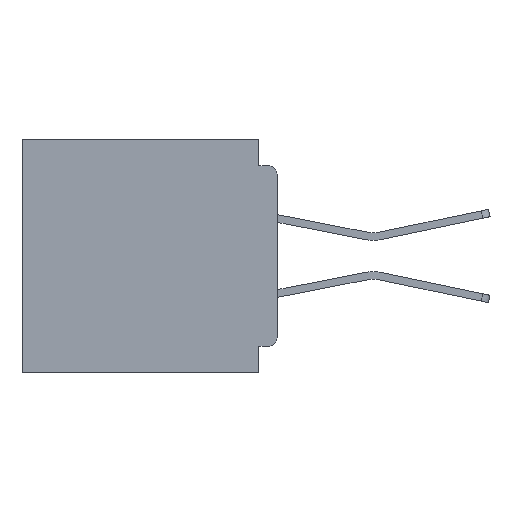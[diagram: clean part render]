
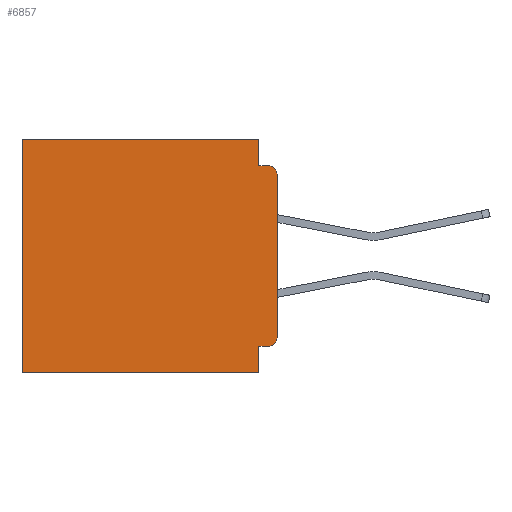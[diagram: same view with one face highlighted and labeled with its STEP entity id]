
A CAD part, left-side view. The second image highlights one B-rep face of the part: STEP entity #6857.
In plain terms, the highlighted planar face has unit normal (-1, 0, 0).
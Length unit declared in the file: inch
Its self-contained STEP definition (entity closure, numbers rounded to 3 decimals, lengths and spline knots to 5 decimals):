
#730 = LINE ( 'NONE', #44997, #26693 ) ;
#810 = VERTEX_POINT ( 'NONE', #28560 ) ;
#841 = EDGE_CURVE ( 'NONE', #22364, #8738, #36034, .T. ) ;
#1111 = AXIS2_PLACEMENT_3D ( 'NONE', #43485, #5299, #29916 ) ;
#1698 = ORIENTED_EDGE ( 'NONE', *, *, #16101, .T. ) ;
#1900 = DIRECTION ( 'NONE',  ( 0., 1., 0. ) ) ;
#2054 = CARTESIAN_POINT ( 'NONE',  ( 0.3, 0.031, 0. ) ) ;
#2116 = EDGE_CURVE ( 'NONE', #8738, #43184, #38074, .T. ) ;
#2700 = LINE ( 'NONE', #23927, #32981 ) ;
#2707 = DIRECTION ( 'NONE',  ( 0., 0., -1. ) ) ;
#3370 = CARTESIAN_POINT ( 'NONE',  ( 0.3, 0.031, -0.355 ) ) ;
#4194 = VERTEX_POINT ( 'NONE', #29689 ) ;
#4697 = VERTEX_POINT ( 'NONE', #42580 ) ;
#5299 = DIRECTION ( 'NONE',  ( 1., 0., 0. ) ) ;
#6207 = ORIENTED_EDGE ( 'NONE', *, *, #26114, .T. ) ;
#6353 = EDGE_CURVE ( 'NONE', #810, #29096, #37275, .T. ) ;
#6642 = EDGE_CURVE ( 'NONE', #4697, #36173, #26437, .T. ) ;
#6857 = ADVANCED_FACE ( 'NONE', ( #16553 ), #26431, .F. ) ;
#7925 = DIRECTION ( 'NONE',  ( 0., 0., -1. ) ) ;
#8738 = VERTEX_POINT ( 'NONE', #25829 ) ;
#8874 = CARTESIAN_POINT ( 'NONE',  ( 0.3, 0.015, -0.06 ) ) ;
#9277 = EDGE_CURVE ( 'NONE', #29096, #4697, #17986, .T. ) ;
#9750 = CARTESIAN_POINT ( 'NONE',  ( 0.3, 0.015, -0.34 ) ) ;
#10229 = ORIENTED_EDGE ( 'NONE', *, *, #28283, .F. ) ;
#10292 = DIRECTION ( 'NONE',  ( 0., 1., 0. ) ) ;
#12437 = DIRECTION ( 'NONE',  ( 0., 0., -1. ) ) ;
#13317 = DIRECTION ( 'NONE',  ( 0., 0., -1. ) ) ;
#15151 = VECTOR ( 'NONE', #23886, 39.37008 ) ;
#15288 = CARTESIAN_POINT ( 'NONE',  ( 0.3, 0.437, 0. ) ) ;
#16058 = CARTESIAN_POINT ( 'NONE',  ( 0.3, 0., -0.355 ) ) ;
#16101 = EDGE_CURVE ( 'NONE', #22364, #39197, #730, .T. ) ;
#16553 = FACE_OUTER_BOUND ( 'NONE', #22328, .T. ) ;
#17986 = LINE ( 'NONE', #32623, #27230 ) ;
#18649 = VECTOR ( 'NONE', #29374, 39.37008 ) ;
#18813 = VECTOR ( 'NONE', #1900, 39.37008 ) ;
#18898 = CARTESIAN_POINT ( 'NONE',  ( 0.3, 0.437, -0.4 ) ) ;
#19289 = AXIS2_PLACEMENT_3D ( 'NONE', #8874, #33376, #12437 ) ;
#19544 = ORIENTED_EDGE ( 'NONE', *, *, #841, .F. ) ;
#22328 = EDGE_LOOP ( 'NONE', ( #10229, #6207, #41476, #19544, #1698, #33990, #35328, #25361, #26263, #43523 ) ) ;
#22364 = VERTEX_POINT ( 'NONE', #30848 ) ;
#23886 = DIRECTION ( 'NONE',  ( 0., 0., -1. ) ) ;
#23927 = CARTESIAN_POINT ( 'NONE',  ( 0.3, 0.437, -0.4 ) ) ;
#25361 = ORIENTED_EDGE ( 'NONE', *, *, #9277, .F. ) ;
#25603 = LINE ( 'NONE', #41133, #15151 ) ;
#25829 = CARTESIAN_POINT ( 'NONE',  ( 0.3, 0.031, -0.045 ) ) ;
#26114 = EDGE_CURVE ( 'NONE', #42092, #43184, #34357, .T. ) ;
#26263 = ORIENTED_EDGE ( 'NONE', *, *, #6353, .F. ) ;
#26431 = PLANE ( 'NONE',  #1111 ) ;
#26437 = LINE ( 'NONE', #38382, #34514 ) ;
#26693 = VECTOR ( 'NONE', #10292, 39.37008 ) ;
#26800 = DIRECTION ( 'NONE',  ( 0., -1., 0. ) ) ;
#27230 = VECTOR ( 'NONE', #7925, 39.37008 ) ;
#28283 = EDGE_CURVE ( 'NONE', #42092, #4194, #25603, .T. ) ;
#28560 = CARTESIAN_POINT ( 'NONE',  ( 0.3, 0.015, -0.355 ) ) ;
#28895 = VECTOR ( 'NONE', #26800, 39.37008 ) ;
#28956 = EDGE_CURVE ( 'NONE', #810, #4194, #35257, .T. ) ;
#29096 = VERTEX_POINT ( 'NONE', #3370 ) ;
#29374 = DIRECTION ( 'NONE',  ( 0., 0., -1. ) ) ;
#29689 = CARTESIAN_POINT ( 'NONE',  ( 0.3, 0., -0.34 ) ) ;
#29916 = DIRECTION ( 'NONE',  ( 0., 0., -1. ) ) ;
#30282 = EDGE_CURVE ( 'NONE', #39197, #36173, #2700, .T. ) ;
#30848 = CARTESIAN_POINT ( 'NONE',  ( 0.3, 0.031, 0. ) ) ;
#32623 = CARTESIAN_POINT ( 'NONE',  ( 0.3, 0.031, -0.4 ) ) ;
#32981 = VECTOR ( 'NONE', #2707, 39.37008 ) ;
#33376 = DIRECTION ( 'NONE',  ( -1., 0., 0. ) ) ;
#33990 = ORIENTED_EDGE ( 'NONE', *, *, #30282, .T. ) ;
#34245 = DIRECTION ( 'NONE',  ( -1., 0., 0. ) ) ;
#34357 = CIRCLE ( 'NONE', #19289, 0.015 ) ;
#34514 = VECTOR ( 'NONE', #41859, 39.37008 ) ;
#35257 = CIRCLE ( 'NONE', #44002, 0.015 ) ;
#35328 = ORIENTED_EDGE ( 'NONE', *, *, #6642, .F. ) ;
#36034 = LINE ( 'NONE', #2054, #18649 ) ;
#36173 = VERTEX_POINT ( 'NONE', #18898 ) ;
#36722 = CARTESIAN_POINT ( 'NONE',  ( 0.3, 0.015, -0.045 ) ) ;
#37275 = LINE ( 'NONE', #16058, #18813 ) ;
#37566 = CARTESIAN_POINT ( 'NONE',  ( 0.3, 0., -0.045 ) ) ;
#38074 = LINE ( 'NONE', #37566, #28895 ) ;
#38382 = CARTESIAN_POINT ( 'NONE',  ( 0.3, 0., -0.4 ) ) ;
#39197 = VERTEX_POINT ( 'NONE', #15288 ) ;
#41133 = CARTESIAN_POINT ( 'NONE',  ( 0.3, 0., -0.4 ) ) ;
#41476 = ORIENTED_EDGE ( 'NONE', *, *, #2116, .F. ) ;
#41859 = DIRECTION ( 'NONE',  ( 0., 1., 0. ) ) ;
#42092 = VERTEX_POINT ( 'NONE', #44749 ) ;
#42580 = CARTESIAN_POINT ( 'NONE',  ( 0.3, 0.031, -0.4 ) ) ;
#43184 = VERTEX_POINT ( 'NONE', #36722 ) ;
#43485 = CARTESIAN_POINT ( 'NONE',  ( 0.3, 0., -0.4 ) ) ;
#43523 = ORIENTED_EDGE ( 'NONE', *, *, #28956, .T. ) ;
#44002 = AXIS2_PLACEMENT_3D ( 'NONE', #9750, #34245, #13317 ) ;
#44749 = CARTESIAN_POINT ( 'NONE',  ( 0.3, 0., -0.06 ) ) ;
#44997 = CARTESIAN_POINT ( 'NONE',  ( 0.3, 0., 0. ) ) ;
